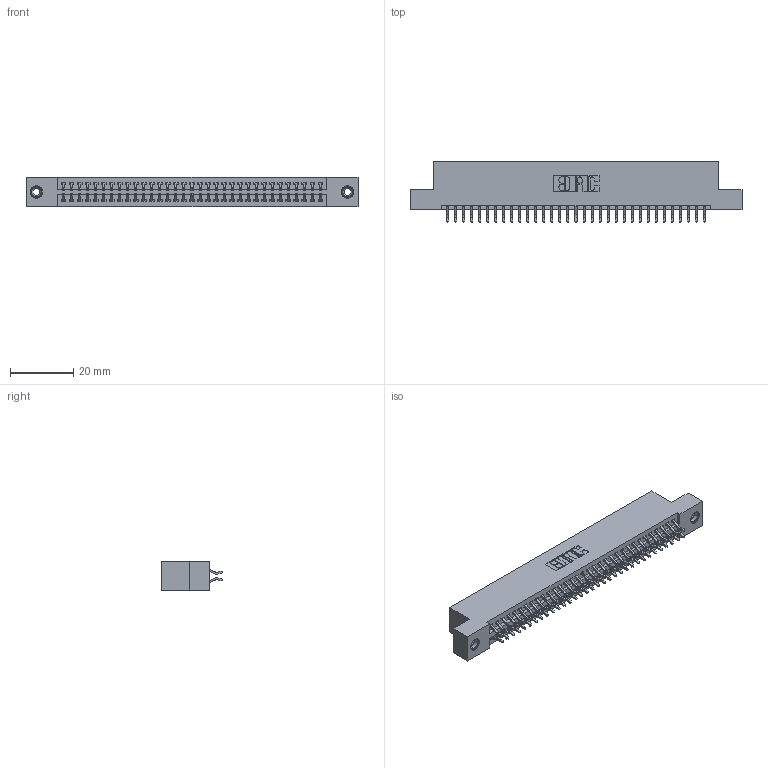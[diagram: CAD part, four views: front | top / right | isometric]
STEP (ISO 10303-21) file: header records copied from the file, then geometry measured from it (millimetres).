
FILE_DESCRIPTION (( 'STEP AP203' ), '1' );
FILE_NAME ('395-066-556-208.STEP', '2019-10-23T21:16:31', ( '' ), ( '' ), 'SwSTEP 2.0', 'SolidWorks 2016', '' );
FILE_SCHEMA (( 'CONFIG_CONTROL_DESIGN' ));
Length unit declared in the file: inch
Products named in the file (4): 345 Part_Flush Mounting Lugs - 0.156 Dia-TI; 345-292-001_556 Tail; 345-250-001_345-250-003-102; 395-066-556-208
Assembly tree (69 placements, depth 2):
  395-066-556-208
    345 Part_Flush Mounting Lugs - 0.156 Dia-TI
    345-292-001_556 Tail  x66
    345-250-001_345-250-003-102  x2
Bounding box: 105.03 x 19.24 x 9.4 mm (x, y, z)
Volume: 10110 mm3; surface area: 14725.6 mm2
Topology: 69 solids, 69 shells, 3882 faces, 11499 edges, 7570 vertices
Faces by surface type: plane 2554, cylinder 1312, cone 12, torus 4
Entity records: 28510 total; most frequent: CARTESIAN_POINT 4783, ORIENTED_EDGE 4698, DIRECTION 4243, EDGE_CURVE 2349, VECTOR 2057, LINE 2057, VERTEX_POINT 1560, AXIS2_PLACEMENT_3D 1093
